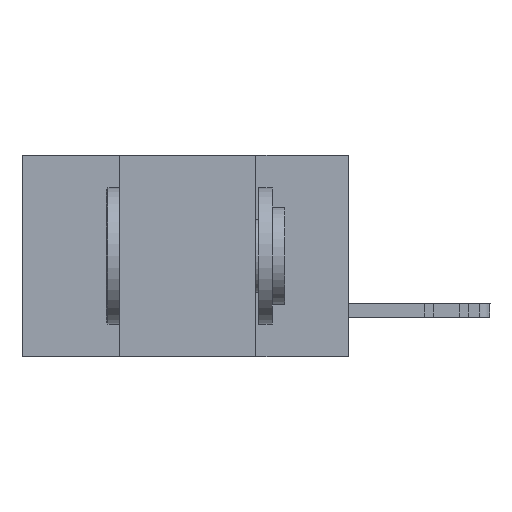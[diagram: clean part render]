
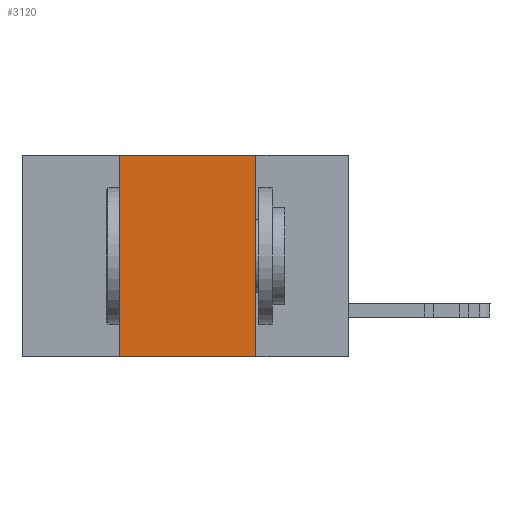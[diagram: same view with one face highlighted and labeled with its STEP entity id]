
A CAD part, left-side view. The second image highlights one B-rep face of the part: STEP entity #3120.
In plain terms, the highlighted planar face has unit normal (-1, 0, 0).
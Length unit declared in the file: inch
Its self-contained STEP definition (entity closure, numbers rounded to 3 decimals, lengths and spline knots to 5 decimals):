
#1175 = VERTEX_POINT ( 'NONE', #6498 ) ;
#3120 = ADVANCED_FACE ( 'NONE', ( #5964 ), #12445, .F. ) ;
#3293 = AXIS2_PLACEMENT_3D ( 'NONE', #9921, #9803, #9593 ) ;
#3802 = CARTESIAN_POINT ( 'NONE',  ( 0., 0.42, -0.37 ) ) ;
#4473 = VECTOR ( 'NONE', #6436, 39.37008 ) ;
#5128 = VECTOR ( 'NONE', #8194, 39.37008 ) ;
#5877 = VERTEX_POINT ( 'NONE', #7789 ) ;
#5964 = FACE_OUTER_BOUND ( 'NONE', #6192, .T. ) ;
#6192 = EDGE_LOOP ( 'NONE', ( #6272, #17293, #12528, #23799 ) ) ;
#6272 = ORIENTED_EDGE ( 'NONE', *, *, #7543, .F. ) ;
#6398 = LINE ( 'NONE', #19127, #22659 ) ;
#6436 = DIRECTION ( 'NONE',  ( 0., -1., 0. ) ) ;
#6498 = CARTESIAN_POINT ( 'NONE',  ( 0., 0.42, 0. ) ) ;
#6700 = DIRECTION ( 'NONE',  ( 0., 0., 1. ) ) ;
#7543 = EDGE_CURVE ( 'NONE', #5877, #13482, #21159, .T. ) ;
#7688 = DIRECTION ( 'NONE',  ( 0., 0., -1. ) ) ;
#7789 = CARTESIAN_POINT ( 'NONE',  ( 0., 0.17, 0. ) ) ;
#7976 = CARTESIAN_POINT ( 'NONE',  ( 0., 0.17, -0.37 ) ) ;
#8194 = DIRECTION ( 'NONE',  ( 0., -1., 0. ) ) ;
#9593 = DIRECTION ( 'NONE',  ( 0., 0., -1. ) ) ;
#9803 = DIRECTION ( 'NONE',  ( 1., 0., 0. ) ) ;
#9921 = CARTESIAN_POINT ( 'NONE',  ( 0., 0.6, 0. ) ) ;
#10064 = LINE ( 'NONE', #18790, #4473 ) ;
#12009 = LINE ( 'NONE', #18394, #5128 ) ;
#12445 = PLANE ( 'NONE',  #3293 ) ;
#12528 = ORIENTED_EDGE ( 'NONE', *, *, #13153, .F. ) ;
#13153 = EDGE_CURVE ( 'NONE', #19484, #1175, #6398, .T. ) ;
#13482 = VERTEX_POINT ( 'NONE', #16558 ) ;
#16558 = CARTESIAN_POINT ( 'NONE',  ( 0., 0.17, -0.37 ) ) ;
#17293 = ORIENTED_EDGE ( 'NONE', *, *, #17809, .F. ) ;
#17809 = EDGE_CURVE ( 'NONE', #1175, #5877, #12009, .T. ) ;
#18394 = CARTESIAN_POINT ( 'NONE',  ( 0., 0.6, 0. ) ) ;
#18790 = CARTESIAN_POINT ( 'NONE',  ( 0., 0.6, -0.37 ) ) ;
#19127 = CARTESIAN_POINT ( 'NONE',  ( 0., 0.42, -0.37 ) ) ;
#19484 = VERTEX_POINT ( 'NONE', #3802 ) ;
#21159 = LINE ( 'NONE', #7976, #25726 ) ;
#21590 = EDGE_CURVE ( 'NONE', #19484, #13482, #10064, .T. ) ;
#22659 = VECTOR ( 'NONE', #6700, 39.37008 ) ;
#23799 = ORIENTED_EDGE ( 'NONE', *, *, #21590, .T. ) ;
#25726 = VECTOR ( 'NONE', #7688, 39.37008 ) ;
